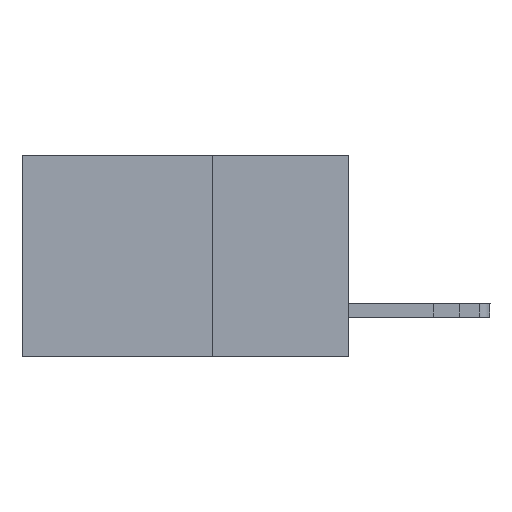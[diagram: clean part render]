
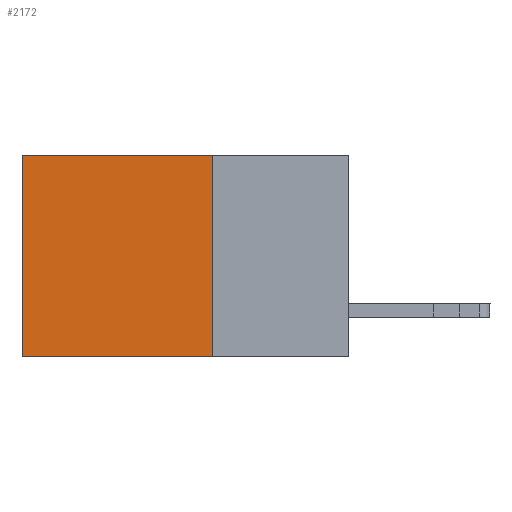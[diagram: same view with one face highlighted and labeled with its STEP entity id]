
A CAD part, left-side view. The second image highlights one B-rep face of the part: STEP entity #2172.
In plain terms, the highlighted planar face has unit normal (-1, 0, 0).
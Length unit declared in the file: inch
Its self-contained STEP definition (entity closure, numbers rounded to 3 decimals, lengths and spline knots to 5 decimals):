
#41 = EDGE_CURVE ( 'NONE', #2494, #144, #5254, .T. ) ;
#73 = EDGE_CURVE ( 'NONE', #10373, #2494, #5830, .T. ) ;
#144 = VERTEX_POINT ( 'NONE', #11506 ) ;
#989 = DIRECTION ( 'NONE',  ( 0., 1., 0. ) ) ;
#1214 = EDGE_LOOP ( 'NONE', ( #2623, #8603, #8043, #11103 ) ) ;
#1441 = LINE ( 'NONE', #9451, #5356 ) ;
#1889 = LINE ( 'NONE', #7616, #11519 ) ;
#1909 = DIRECTION ( 'NONE',  ( 1., 0., 0. ) ) ;
#2092 = CARTESIAN_POINT ( 'NONE',  ( 0.298, 0.6, 0. ) ) ;
#2172 = ADVANCED_FACE ( 'NONE', ( #8452 ), #8581, .F. ) ;
#2494 = VERTEX_POINT ( 'NONE', #6194 ) ;
#2623 = ORIENTED_EDGE ( 'NONE', *, *, #7471, .T. ) ;
#2748 = DIRECTION ( 'NONE',  ( 0., 0., -1. ) ) ;
#3305 = VERTEX_POINT ( 'NONE', #2092 ) ;
#3442 = AXIS2_PLACEMENT_3D ( 'NONE', #7478, #1909, #9382 ) ;
#4960 = CARTESIAN_POINT ( 'NONE',  ( 0.298, 0.25, -0.37 ) ) ;
#5254 = LINE ( 'NONE', #4960, #7433 ) ;
#5356 = VECTOR ( 'NONE', #989, 39.37008 ) ;
#5830 = LINE ( 'NONE', #11149, #7141 ) ;
#6194 = CARTESIAN_POINT ( 'NONE',  ( 0.298, 0.25, -0.37 ) ) ;
#6718 = DIRECTION ( 'NONE',  ( 0., 0., -1. ) ) ;
#7141 = VECTOR ( 'NONE', #2748, 39.37008 ) ;
#7433 = VECTOR ( 'NONE', #7667, 39.37008 ) ;
#7471 = EDGE_CURVE ( 'NONE', #3305, #144, #1889, .T. ) ;
#7478 = CARTESIAN_POINT ( 'NONE',  ( 0.298, 0.25, 0. ) ) ;
#7616 = CARTESIAN_POINT ( 'NONE',  ( 0.298, 0.6, 0. ) ) ;
#7667 = DIRECTION ( 'NONE',  ( 0., 1., 0. ) ) ;
#8043 = ORIENTED_EDGE ( 'NONE', *, *, #73, .F. ) ;
#8082 = EDGE_CURVE ( 'NONE', #10373, #3305, #1441, .T. ) ;
#8452 = FACE_OUTER_BOUND ( 'NONE', #1214, .T. ) ;
#8581 = PLANE ( 'NONE',  #3442 ) ;
#8603 = ORIENTED_EDGE ( 'NONE', *, *, #41, .F. ) ;
#9382 = DIRECTION ( 'NONE',  ( 0., 0., -1. ) ) ;
#9451 = CARTESIAN_POINT ( 'NONE',  ( 0.298, 0.25, 0. ) ) ;
#10373 = VERTEX_POINT ( 'NONE', #11326 ) ;
#11103 = ORIENTED_EDGE ( 'NONE', *, *, #8082, .T. ) ;
#11149 = CARTESIAN_POINT ( 'NONE',  ( 0.298, 0.25, 0. ) ) ;
#11326 = CARTESIAN_POINT ( 'NONE',  ( 0.298, 0.25, 0. ) ) ;
#11506 = CARTESIAN_POINT ( 'NONE',  ( 0.298, 0.6, -0.37 ) ) ;
#11519 = VECTOR ( 'NONE', #6718, 39.37008 ) ;
